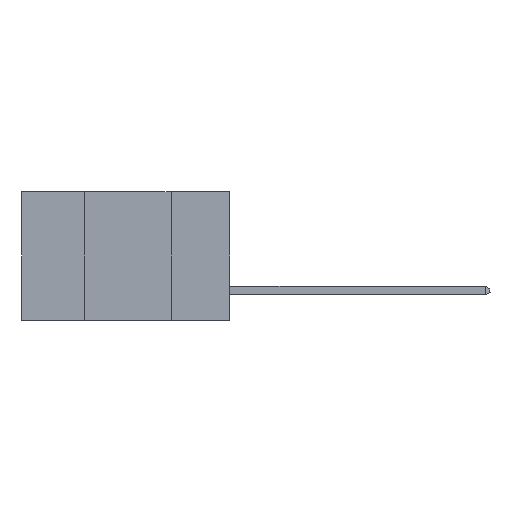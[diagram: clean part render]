
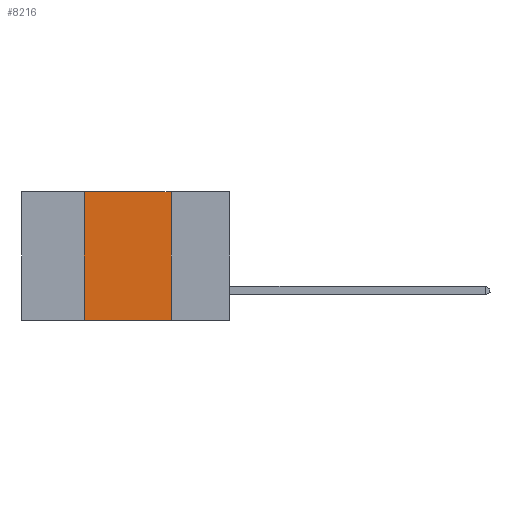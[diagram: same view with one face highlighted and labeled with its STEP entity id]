
A CAD part, left-side view. The second image highlights one B-rep face of the part: STEP entity #8216.
In plain terms, the highlighted planar face has unit normal (-1, 0, 0).
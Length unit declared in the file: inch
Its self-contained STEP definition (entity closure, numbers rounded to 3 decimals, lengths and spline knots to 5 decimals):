
#525 = ORIENTED_EDGE ( 'NONE', *, *, #13226, .F. ) ;
#712 = LINE ( 'NONE', #9729, #15482 ) ;
#1086 = DIRECTION ( 'NONE',  ( 0., -1., 0. ) ) ;
#1933 = CARTESIAN_POINT ( 'NONE',  ( 0., 0.6, -0.37 ) ) ;
#2124 = EDGE_CURVE ( 'NONE', #9265, #15927, #17342, .T. ) ;
#2390 = DIRECTION ( 'NONE',  ( 1., 0., 0. ) ) ;
#2546 = VERTEX_POINT ( 'NONE', #7973 ) ;
#2805 = DIRECTION ( 'NONE',  ( 0., 0., 1. ) ) ;
#3692 = ORIENTED_EDGE ( 'NONE', *, *, #7074, .F. ) ;
#6157 = ORIENTED_EDGE ( 'NONE', *, *, #2124, .T. ) ;
#7074 = EDGE_CURVE ( 'NONE', #9265, #2546, #16501, .T. ) ;
#7464 = VECTOR ( 'NONE', #2805, 39.37008 ) ;
#7872 = PLANE ( 'NONE',  #14736 ) ;
#7973 = CARTESIAN_POINT ( 'NONE',  ( 0., 0.42, 0. ) ) ;
#8216 = ADVANCED_FACE ( 'NONE', ( #11375 ), #7872, .F. ) ;
#8499 = EDGE_LOOP ( 'NONE', ( #525, #8666, #3692, #6157 ) ) ;
#8666 = ORIENTED_EDGE ( 'NONE', *, *, #9522, .F. ) ;
#9265 = VERTEX_POINT ( 'NONE', #10273 ) ;
#9522 = EDGE_CURVE ( 'NONE', #2546, #11236, #712, .T. ) ;
#9729 = CARTESIAN_POINT ( 'NONE',  ( 0., 0.6, 0. ) ) ;
#10273 = CARTESIAN_POINT ( 'NONE',  ( 0., 0.42, -0.37 ) ) ;
#10455 = DIRECTION ( 'NONE',  ( 0., -1., 0. ) ) ;
#10745 = VECTOR ( 'NONE', #11442, 39.37008 ) ;
#11215 = CARTESIAN_POINT ( 'NONE',  ( 0., 0.42, 0. ) ) ;
#11236 = VERTEX_POINT ( 'NONE', #17541 ) ;
#11375 = FACE_OUTER_BOUND ( 'NONE', #8499, .T. ) ;
#11385 = CARTESIAN_POINT ( 'NONE',  ( 0., 0.17, 0. ) ) ;
#11442 = DIRECTION ( 'NONE',  ( 0., 0., -1. ) ) ;
#11622 = LINE ( 'NONE', #11385, #10745 ) ;
#13226 = EDGE_CURVE ( 'NONE', #11236, #15927, #11622, .T. ) ;
#14722 = VECTOR ( 'NONE', #10455, 39.37008 ) ;
#14736 = AXIS2_PLACEMENT_3D ( 'NONE', #15084, #2390, #14952 ) ;
#14952 = DIRECTION ( 'NONE',  ( 0., 0., -1. ) ) ;
#15084 = CARTESIAN_POINT ( 'NONE',  ( 0., 0.6, 0. ) ) ;
#15482 = VECTOR ( 'NONE', #1086, 39.37008 ) ;
#15927 = VERTEX_POINT ( 'NONE', #16394 ) ;
#16394 = CARTESIAN_POINT ( 'NONE',  ( 0., 0.17, -0.37 ) ) ;
#16501 = LINE ( 'NONE', #11215, #7464 ) ;
#17342 = LINE ( 'NONE', #1933, #14722 ) ;
#17541 = CARTESIAN_POINT ( 'NONE',  ( 0., 0.17, 0. ) ) ;
